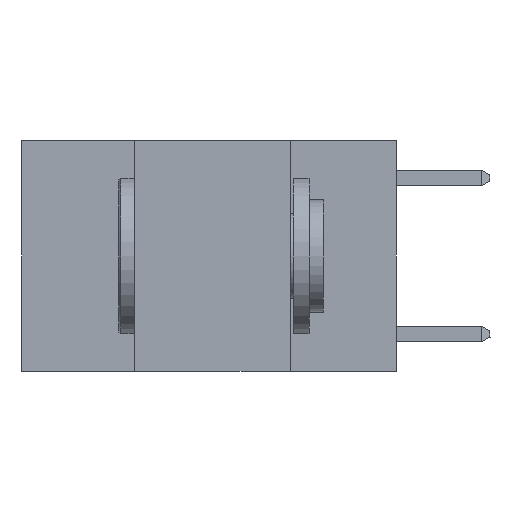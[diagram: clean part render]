
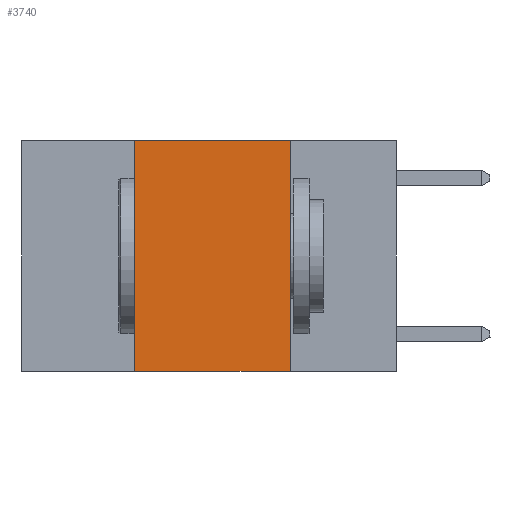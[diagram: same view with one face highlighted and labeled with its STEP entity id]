
A CAD part, left-side view. The second image highlights one B-rep face of the part: STEP entity #3740.
In plain terms, the highlighted planar face has unit normal (-1, 0, 0).
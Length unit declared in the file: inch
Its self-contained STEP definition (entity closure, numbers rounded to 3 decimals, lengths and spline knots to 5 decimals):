
#487 = EDGE_CURVE ( 'NONE', #9798, #3657, #12391, .T. ) ;
#595 = CARTESIAN_POINT ( 'NONE',  ( 0., 0.17, 0. ) ) ;
#1422 = EDGE_CURVE ( 'NONE', #3396, #2673, #3797, .T. ) ;
#1727 = DIRECTION ( 'NONE',  ( 0., 0., -1. ) ) ;
#2465 = EDGE_CURVE ( 'NONE', #2673, #3657, #6059, .T. ) ;
#2673 = VERTEX_POINT ( 'NONE', #6166 ) ;
#3023 = VECTOR ( 'NONE', #10566, 39.37008 ) ;
#3396 = VERTEX_POINT ( 'NONE', #7905 ) ;
#3657 = VERTEX_POINT ( 'NONE', #10761 ) ;
#3740 = ADVANCED_FACE ( 'NONE', ( #4432 ), #4143, .F. ) ;
#3797 = LINE ( 'NONE', #12923, #13012 ) ;
#4112 = EDGE_CURVE ( 'NONE', #9798, #3396, #6097, .T. ) ;
#4143 = PLANE ( 'NONE',  #10563 ) ;
#4432 = FACE_OUTER_BOUND ( 'NONE', #10709, .T. ) ;
#4930 = CARTESIAN_POINT ( 'NONE',  ( 0., 0.42, 0. ) ) ;
#5171 = DIRECTION ( 'NONE',  ( 0., -1., 0. ) ) ;
#5642 = CARTESIAN_POINT ( 'NONE',  ( 0., 0.6, -0.37 ) ) ;
#6059 = LINE ( 'NONE', #595, #9045 ) ;
#6097 = LINE ( 'NONE', #4930, #3023 ) ;
#6166 = CARTESIAN_POINT ( 'NONE',  ( 0., 0.17, 0. ) ) ;
#7768 = ORIENTED_EDGE ( 'NONE', *, *, #487, .T. ) ;
#7905 = CARTESIAN_POINT ( 'NONE',  ( 0., 0.42, 0. ) ) ;
#8215 = ORIENTED_EDGE ( 'NONE', *, *, #1422, .F. ) ;
#8651 = DIRECTION ( 'NONE',  ( 1., 0., 0. ) ) ;
#8754 = DIRECTION ( 'NONE',  ( 0., 0., -1. ) ) ;
#9045 = VECTOR ( 'NONE', #8754, 39.37008 ) ;
#9798 = VERTEX_POINT ( 'NONE', #12011 ) ;
#9803 = ORIENTED_EDGE ( 'NONE', *, *, #4112, .F. ) ;
#10563 = AXIS2_PLACEMENT_3D ( 'NONE', #13021, #8651, #1727 ) ;
#10566 = DIRECTION ( 'NONE',  ( 0., 0., 1. ) ) ;
#10709 = EDGE_LOOP ( 'NONE', ( #14616, #8215, #9803, #7768 ) ) ;
#10761 = CARTESIAN_POINT ( 'NONE',  ( 0., 0.17, -0.37 ) ) ;
#11385 = DIRECTION ( 'NONE',  ( 0., -1., 0. ) ) ;
#12011 = CARTESIAN_POINT ( 'NONE',  ( 0., 0.42, -0.37 ) ) ;
#12391 = LINE ( 'NONE', #5642, #12718 ) ;
#12718 = VECTOR ( 'NONE', #11385, 39.37008 ) ;
#12923 = CARTESIAN_POINT ( 'NONE',  ( 0., 0.6, 0. ) ) ;
#13012 = VECTOR ( 'NONE', #5171, 39.37008 ) ;
#13021 = CARTESIAN_POINT ( 'NONE',  ( 0., 0.6, 0. ) ) ;
#14616 = ORIENTED_EDGE ( 'NONE', *, *, #2465, .F. ) ;
